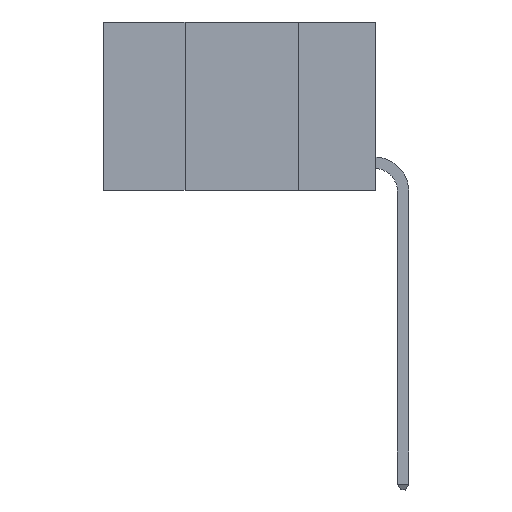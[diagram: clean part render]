
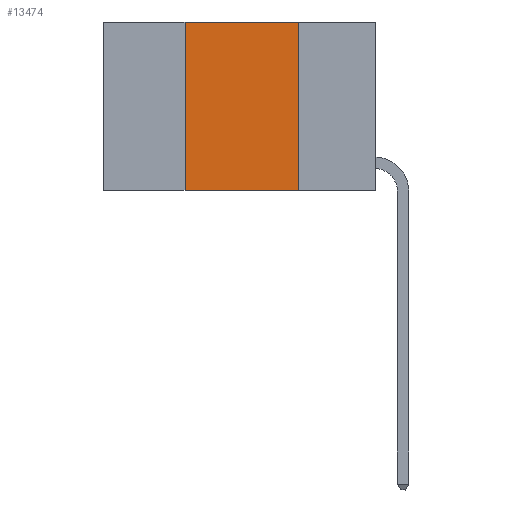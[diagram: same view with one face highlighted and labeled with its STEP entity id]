
A CAD part, left-side view. The second image highlights one B-rep face of the part: STEP entity #13474.
In plain terms, the highlighted planar face has unit normal (-1, 0, 0).
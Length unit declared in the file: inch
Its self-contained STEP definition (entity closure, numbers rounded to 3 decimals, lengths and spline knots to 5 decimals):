
#319 = CARTESIAN_POINT ( 'NONE',  ( 0., 0.42, -0.37 ) ) ;
#406 = EDGE_CURVE ( 'NONE', #24702, #22411, #24440, .T. ) ;
#1739 = PLANE ( 'NONE',  #11821 ) ;
#3263 = ORIENTED_EDGE ( 'NONE', *, *, #25405, .T. ) ;
#3673 = VECTOR ( 'NONE', #15869, 39.37008 ) ;
#3774 = DIRECTION ( 'NONE',  ( 1., 0., 0. ) ) ;
#4385 = DIRECTION ( 'NONE',  ( 0., 0., 1. ) ) ;
#5192 = CARTESIAN_POINT ( 'NONE',  ( 0., 0.42, 0. ) ) ;
#6249 = DIRECTION ( 'NONE',  ( 0., -1., 0. ) ) ;
#6706 = EDGE_LOOP ( 'NONE', ( #20674, #20724, #22875, #3263 ) ) ;
#7161 = FACE_OUTER_BOUND ( 'NONE', #6706, .T. ) ;
#8781 = EDGE_CURVE ( 'NONE', #13665, #24702, #16781, .T. ) ;
#9809 = VERTEX_POINT ( 'NONE', #17779 ) ;
#10335 = CARTESIAN_POINT ( 'NONE',  ( 0., 0.42, 0. ) ) ;
#11564 = VECTOR ( 'NONE', #4385, 39.37008 ) ;
#11821 = AXIS2_PLACEMENT_3D ( 'NONE', #13673, #3774, #17652 ) ;
#13250 = VECTOR ( 'NONE', #6249, 39.37008 ) ;
#13474 = ADVANCED_FACE ( 'NONE', ( #7161 ), #1739, .F. ) ;
#13665 = VERTEX_POINT ( 'NONE', #319 ) ;
#13673 = CARTESIAN_POINT ( 'NONE',  ( 0., 0.6, 0. ) ) ;
#14243 = CARTESIAN_POINT ( 'NONE',  ( 0., 0.17, 0. ) ) ;
#14390 = CARTESIAN_POINT ( 'NONE',  ( 0., 0.17, 0. ) ) ;
#14907 = EDGE_CURVE ( 'NONE', #22411, #9809, #19536, .T. ) ;
#15869 = DIRECTION ( 'NONE',  ( 0., -1., 0. ) ) ;
#16781 = LINE ( 'NONE', #10335, #11564 ) ;
#17652 = DIRECTION ( 'NONE',  ( 0., 0., -1. ) ) ;
#17779 = CARTESIAN_POINT ( 'NONE',  ( 0., 0.17, -0.37 ) ) ;
#19536 = LINE ( 'NONE', #14390, #24213 ) ;
#20674 = ORIENTED_EDGE ( 'NONE', *, *, #14907, .F. ) ;
#20724 = ORIENTED_EDGE ( 'NONE', *, *, #406, .F. ) ;
#21601 = CARTESIAN_POINT ( 'NONE',  ( 0., 0.6, 0. ) ) ;
#22411 = VERTEX_POINT ( 'NONE', #14243 ) ;
#22875 = ORIENTED_EDGE ( 'NONE', *, *, #8781, .F. ) ;
#23800 = CARTESIAN_POINT ( 'NONE',  ( 0., 0.6, -0.37 ) ) ;
#24194 = LINE ( 'NONE', #23800, #3673 ) ;
#24213 = VECTOR ( 'NONE', #24309, 39.37008 ) ;
#24309 = DIRECTION ( 'NONE',  ( 0., 0., -1. ) ) ;
#24440 = LINE ( 'NONE', #21601, #13250 ) ;
#24702 = VERTEX_POINT ( 'NONE', #5192 ) ;
#25405 = EDGE_CURVE ( 'NONE', #13665, #9809, #24194, .T. ) ;
